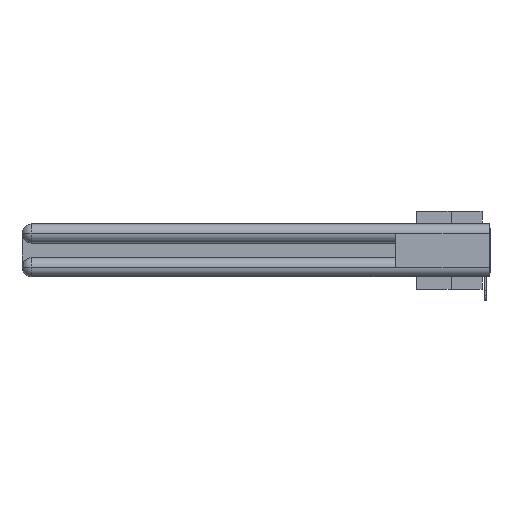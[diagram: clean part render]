
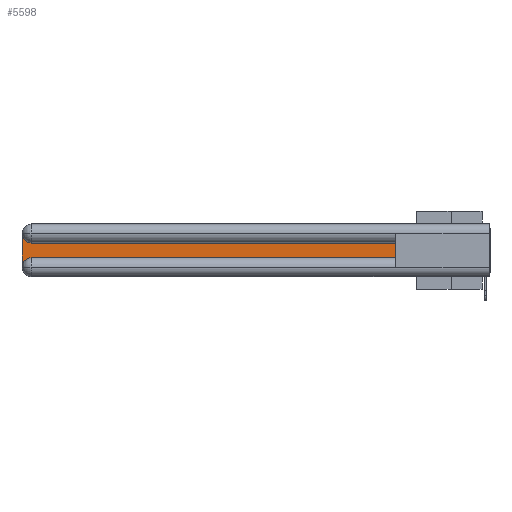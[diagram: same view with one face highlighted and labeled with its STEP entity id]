
A CAD part, left-side view. The second image highlights one B-rep face of the part: STEP entity #5598.
In plain terms, the highlighted planar face has unit normal (-1, 0, 0).
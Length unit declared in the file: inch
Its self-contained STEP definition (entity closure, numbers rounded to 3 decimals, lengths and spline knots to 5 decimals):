
#436 = ORIENTED_EDGE ( 'NONE', *, *, #26126, .T. ) ;
#705 = EDGE_CURVE ( 'NONE', #7098, #7295, #16494, .T. ) ;
#1463 = ORIENTED_EDGE ( 'NONE', *, *, #20138, .T. ) ;
#3078 = PLANE ( 'NONE',  #14707 ) ;
#3449 = DIRECTION ( 'NONE',  ( 0., 0., -1. ) ) ;
#3587 = DIRECTION ( 'NONE',  ( 0., -1., 0. ) ) ;
#3721 = VECTOR ( 'NONE', #3449, 39.37008 ) ;
#3874 = ORIENTED_EDGE ( 'NONE', *, *, #6523, .T. ) ;
#4702 = EDGE_CURVE ( 'NONE', #13775, #7098, #16329, .T. ) ;
#5161 = CARTESIAN_POINT ( 'NONE',  ( 0.075, 3., -0.1225 ) ) ;
#5228 = VECTOR ( 'NONE', #3587, 39.37008 ) ;
#5490 = CARTESIAN_POINT ( 'NONE',  ( 0.075, 0.6, -0.2175 ) ) ;
#5598 = ADVANCED_FACE ( 'NONE', ( #12272 ), #3078, .F. ) ;
#6523 = EDGE_CURVE ( 'NONE', #17668, #27061, #10565, .T. ) ;
#7098 = VERTEX_POINT ( 'NONE', #11424 ) ;
#7295 = VERTEX_POINT ( 'NONE', #14057 ) ;
#7510 = DIRECTION ( 'NONE',  ( 1., 0., 0. ) ) ;
#7547 = DIRECTION ( 'NONE',  ( 0., 0., -1. ) ) ;
#8400 = DIRECTION ( 'NONE',  ( 0., 0., -1. ) ) ;
#10138 = CARTESIAN_POINT ( 'NONE',  ( 0.075, 3., -0.2175 ) ) ;
#10387 = DIRECTION ( 'NONE',  ( 0., 0., 1. ) ) ;
#10565 = LINE ( 'NONE', #28972, #5228 ) ;
#11424 = CARTESIAN_POINT ( 'NONE',  ( 0.075, 2.94, -0.1225 ) ) ;
#11442 = EDGE_LOOP ( 'NONE', ( #15735, #24139, #436, #25097, #3874, #1463 ) ) ;
#11749 = CARTESIAN_POINT ( 'NONE',  ( 0.075, 0.6, -0.1225 ) ) ;
#12272 = FACE_OUTER_BOUND ( 'NONE', #11442, .T. ) ;
#13363 = CARTESIAN_POINT ( 'NONE',  ( 0.075, 0.6, -0.1225 ) ) ;
#13775 = VERTEX_POINT ( 'NONE', #13363 ) ;
#13874 = CARTESIAN_POINT ( 'NONE',  ( 0.075, 2.94, -0.0625 ) ) ;
#14057 = CARTESIAN_POINT ( 'NONE',  ( 0.075, 3., -0.0625 ) ) ;
#14707 = AXIS2_PLACEMENT_3D ( 'NONE', #5161, #19104, #7547 ) ;
#15331 = CARTESIAN_POINT ( 'NONE',  ( 0.075, 2.94, -0.2775 ) ) ;
#15365 = CARTESIAN_POINT ( 'NONE',  ( 0.075, 2.94, -0.2175 ) ) ;
#15735 = ORIENTED_EDGE ( 'NONE', *, *, #4702, .T. ) ;
#16329 = LINE ( 'NONE', #11749, #19457 ) ;
#16381 = DIRECTION ( 'NONE',  ( 0., 0., -1. ) ) ;
#16494 = CIRCLE ( 'NONE', #22668, 0.06 ) ;
#16656 = LINE ( 'NONE', #10138, #3721 ) ;
#16756 = VECTOR ( 'NONE', #10387, 39.37008 ) ;
#17420 = CARTESIAN_POINT ( 'NONE',  ( 0.075, 0.6, -0.2175 ) ) ;
#17484 = EDGE_CURVE ( 'NONE', #28353, #17668, #23832, .T. ) ;
#17668 = VERTEX_POINT ( 'NONE', #15365 ) ;
#19104 = DIRECTION ( 'NONE',  ( 1., 0., 0. ) ) ;
#19253 = CARTESIAN_POINT ( 'NONE',  ( 0.075, 3., -0.2775 ) ) ;
#19457 = VECTOR ( 'NONE', #20795, 39.37008 ) ;
#20138 = EDGE_CURVE ( 'NONE', #27061, #13775, #28053, .T. ) ;
#20795 = DIRECTION ( 'NONE',  ( 0., 1., 0. ) ) ;
#20988 = AXIS2_PLACEMENT_3D ( 'NONE', #15331, #25510, #8400 ) ;
#22668 = AXIS2_PLACEMENT_3D ( 'NONE', #13874, #7510, #16381 ) ;
#23832 = CIRCLE ( 'NONE', #20988, 0.06 ) ;
#24139 = ORIENTED_EDGE ( 'NONE', *, *, #705, .T. ) ;
#25097 = ORIENTED_EDGE ( 'NONE', *, *, #17484, .T. ) ;
#25510 = DIRECTION ( 'NONE',  ( 1., 0., 0. ) ) ;
#26126 = EDGE_CURVE ( 'NONE', #7295, #28353, #16656, .T. ) ;
#27061 = VERTEX_POINT ( 'NONE', #17420 ) ;
#28053 = LINE ( 'NONE', #5490, #16756 ) ;
#28353 = VERTEX_POINT ( 'NONE', #19253 ) ;
#28972 = CARTESIAN_POINT ( 'NONE',  ( 0.075, 0.6, -0.2175 ) ) ;
